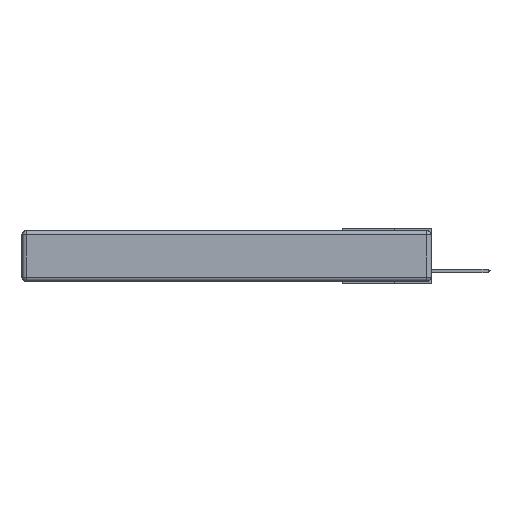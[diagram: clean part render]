
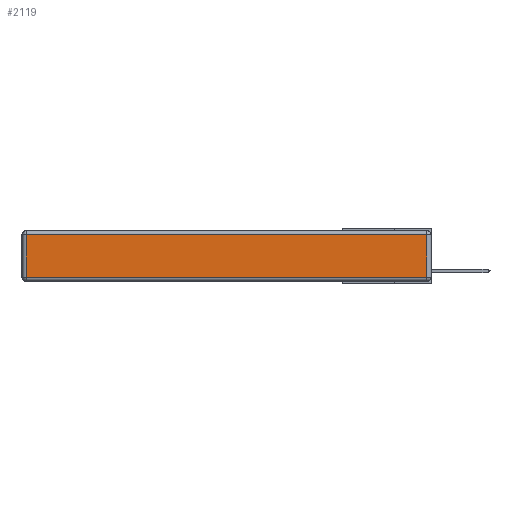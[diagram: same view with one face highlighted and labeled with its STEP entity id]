
A CAD part, left-side view. The second image highlights one B-rep face of the part: STEP entity #2119.
In plain terms, the highlighted planar face has unit normal (-1, 0, 0).
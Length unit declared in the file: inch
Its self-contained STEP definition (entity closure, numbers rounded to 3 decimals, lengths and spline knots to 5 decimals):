
#60 = DIRECTION ( 'NONE',  ( 0., 0., 1. ) ) ;
#530 = VERTEX_POINT ( 'NONE', #16725 ) ;
#604 = LINE ( 'NONE', #5966, #14124 ) ;
#1414 = DIRECTION ( 'NONE',  ( 0., -1., 0. ) ) ;
#1485 = EDGE_CURVE ( 'NONE', #11206, #2790, #7672, .T. ) ;
#1636 = DIRECTION ( 'NONE',  ( 0., 1., 0. ) ) ;
#1870 = ORIENTED_EDGE ( 'NONE', *, *, #1485, .T. ) ;
#2119 = ADVANCED_FACE ( 'NONE', ( #4849 ), #3084, .T. ) ;
#2642 = CARTESIAN_POINT ( 'NONE',  ( 0., 0., -0.313 ) ) ;
#2790 = VERTEX_POINT ( 'NONE', #17961 ) ;
#3009 = EDGE_LOOP ( 'NONE', ( #9415, #1870, #16692, #12329 ) ) ;
#3084 = PLANE ( 'NONE',  #18178 ) ;
#4849 = FACE_OUTER_BOUND ( 'NONE', #3009, .T. ) ;
#5576 = CARTESIAN_POINT ( 'NONE',  ( 0., 2.72, -0.313 ) ) ;
#5966 = CARTESIAN_POINT ( 'NONE',  ( 0., 2.75, -0.03 ) ) ;
#6884 = CARTESIAN_POINT ( 'NONE',  ( 0., 0.03, -0.343 ) ) ;
#7443 = LINE ( 'NONE', #12081, #12103 ) ;
#7672 = LINE ( 'NONE', #6884, #8123 ) ;
#8123 = VECTOR ( 'NONE', #17370, 39.37008 ) ;
#8833 = EDGE_CURVE ( 'NONE', #2790, #530, #604, .T. ) ;
#9415 = ORIENTED_EDGE ( 'NONE', *, *, #10623, .T. ) ;
#10087 = VECTOR ( 'NONE', #1414, 39.37008 ) ;
#10607 = CARTESIAN_POINT ( 'NONE',  ( 0., 0., -0.343 ) ) ;
#10623 = EDGE_CURVE ( 'NONE', #17381, #11206, #14737, .T. ) ;
#11206 = VERTEX_POINT ( 'NONE', #17525 ) ;
#12081 = CARTESIAN_POINT ( 'NONE',  ( 0., 2.72, -0.343 ) ) ;
#12103 = VECTOR ( 'NONE', #15336, 39.37008 ) ;
#12146 = EDGE_CURVE ( 'NONE', #530, #17381, #7443, .T. ) ;
#12329 = ORIENTED_EDGE ( 'NONE', *, *, #12146, .T. ) ;
#13539 = DIRECTION ( 'NONE',  ( -1., 0., 0. ) ) ;
#14124 = VECTOR ( 'NONE', #1636, 39.37008 ) ;
#14737 = LINE ( 'NONE', #2642, #10087 ) ;
#15336 = DIRECTION ( 'NONE',  ( 0., 0., -1. ) ) ;
#16692 = ORIENTED_EDGE ( 'NONE', *, *, #8833, .T. ) ;
#16725 = CARTESIAN_POINT ( 'NONE',  ( 0., 2.72, -0.03 ) ) ;
#17370 = DIRECTION ( 'NONE',  ( 0., 0., 1. ) ) ;
#17381 = VERTEX_POINT ( 'NONE', #5576 ) ;
#17525 = CARTESIAN_POINT ( 'NONE',  ( 0., 0.03, -0.313 ) ) ;
#17961 = CARTESIAN_POINT ( 'NONE',  ( 0., 0.03, -0.03 ) ) ;
#18178 = AXIS2_PLACEMENT_3D ( 'NONE', #10607, #13539, #60 ) ;
